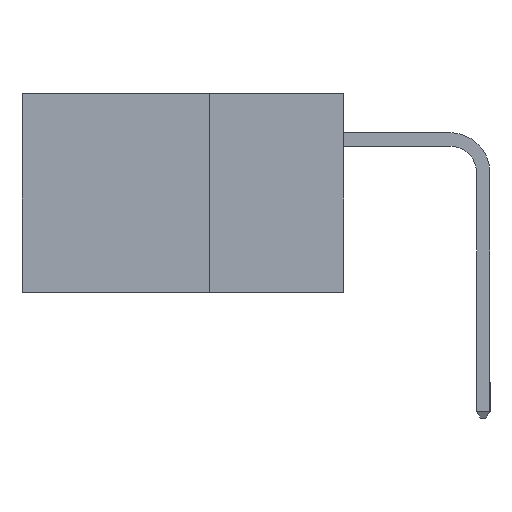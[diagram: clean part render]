
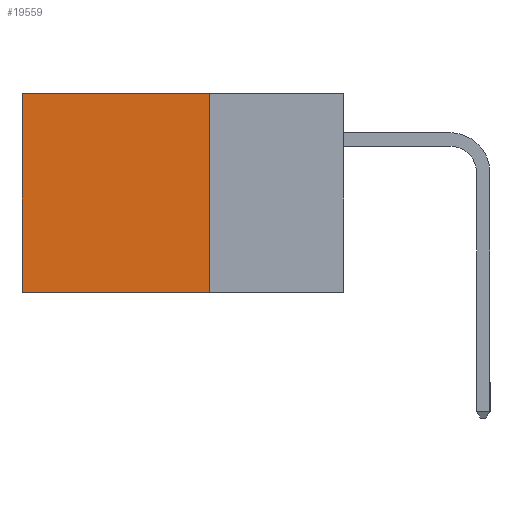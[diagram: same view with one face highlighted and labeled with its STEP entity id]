
A CAD part, left-side view. The second image highlights one B-rep face of the part: STEP entity #19559.
In plain terms, the highlighted planar face has unit normal (-1, 0, 0).
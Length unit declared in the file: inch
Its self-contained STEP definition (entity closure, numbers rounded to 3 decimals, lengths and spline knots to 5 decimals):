
#347 = DIRECTION ( 'NONE',  ( 0., 0., -1. ) ) ;
#478 = VECTOR ( 'NONE', #14629, 39.37008 ) ;
#1188 = EDGE_CURVE ( 'NONE', #18357, #13755, #13858, .T. ) ;
#1604 = LINE ( 'NONE', #10438, #17801 ) ;
#1821 = PLANE ( 'NONE',  #15802 ) ;
#2187 = ORIENTED_EDGE ( 'NONE', *, *, #10909, .T. ) ;
#2426 = VECTOR ( 'NONE', #5169, 39.37008 ) ;
#2488 = DIRECTION ( 'NONE',  ( 0., 1., 0. ) ) ;
#2621 = ORIENTED_EDGE ( 'NONE', *, *, #8274, .T. ) ;
#3672 = CARTESIAN_POINT ( 'NONE',  ( 0.298, 0.25, -0.37 ) ) ;
#4831 = CARTESIAN_POINT ( 'NONE',  ( 0.298, 0.25, 0. ) ) ;
#5084 = CARTESIAN_POINT ( 'NONE',  ( 0.298, 0.25, 0. ) ) ;
#5169 = DIRECTION ( 'NONE',  ( 0., 0., -1. ) ) ;
#5775 = DIRECTION ( 'NONE',  ( 0., 1., 0. ) ) ;
#6014 = FACE_OUTER_BOUND ( 'NONE', #20070, .T. ) ;
#6152 = CARTESIAN_POINT ( 'NONE',  ( 0.298, 0.25, -0.37 ) ) ;
#6327 = VERTEX_POINT ( 'NONE', #14701 ) ;
#7285 = EDGE_CURVE ( 'NONE', #16955, #18357, #10808, .T. ) ;
#7762 = ORIENTED_EDGE ( 'NONE', *, *, #7285, .F. ) ;
#8274 = EDGE_CURVE ( 'NONE', #6327, #13755, #8897, .T. ) ;
#8897 = LINE ( 'NONE', #14611, #478 ) ;
#9837 = DIRECTION ( 'NONE',  ( 1., 0., 0. ) ) ;
#10438 = CARTESIAN_POINT ( 'NONE',  ( 0.298, 0.25, 0. ) ) ;
#10808 = LINE ( 'NONE', #4831, #2426 ) ;
#10909 = EDGE_CURVE ( 'NONE', #16955, #6327, #1604, .T. ) ;
#13755 = VERTEX_POINT ( 'NONE', #17972 ) ;
#13858 = LINE ( 'NONE', #6152, #17053 ) ;
#14011 = CARTESIAN_POINT ( 'NONE',  ( 0.298, 0.25, 0. ) ) ;
#14611 = CARTESIAN_POINT ( 'NONE',  ( 0.298, 0.6, 0. ) ) ;
#14629 = DIRECTION ( 'NONE',  ( 0., 0., -1. ) ) ;
#14701 = CARTESIAN_POINT ( 'NONE',  ( 0.298, 0.6, 0. ) ) ;
#15802 = AXIS2_PLACEMENT_3D ( 'NONE', #5084, #9837, #347 ) ;
#16470 = ORIENTED_EDGE ( 'NONE', *, *, #1188, .F. ) ;
#16955 = VERTEX_POINT ( 'NONE', #14011 ) ;
#17053 = VECTOR ( 'NONE', #2488, 39.37008 ) ;
#17801 = VECTOR ( 'NONE', #5775, 39.37008 ) ;
#17972 = CARTESIAN_POINT ( 'NONE',  ( 0.298, 0.6, -0.37 ) ) ;
#18357 = VERTEX_POINT ( 'NONE', #3672 ) ;
#19559 = ADVANCED_FACE ( 'NONE', ( #6014 ), #1821, .F. ) ;
#20070 = EDGE_LOOP ( 'NONE', ( #2621, #16470, #7762, #2187 ) ) ;
